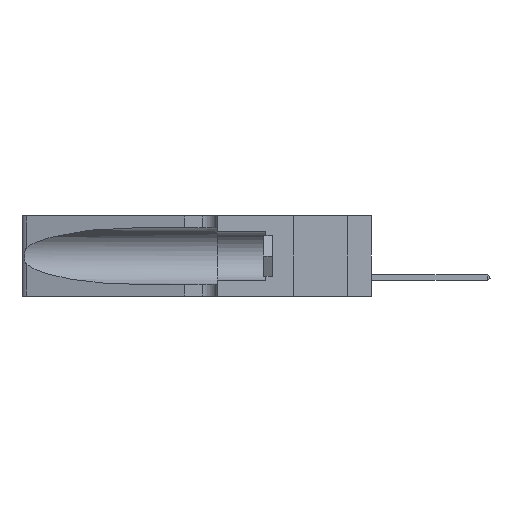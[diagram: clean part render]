
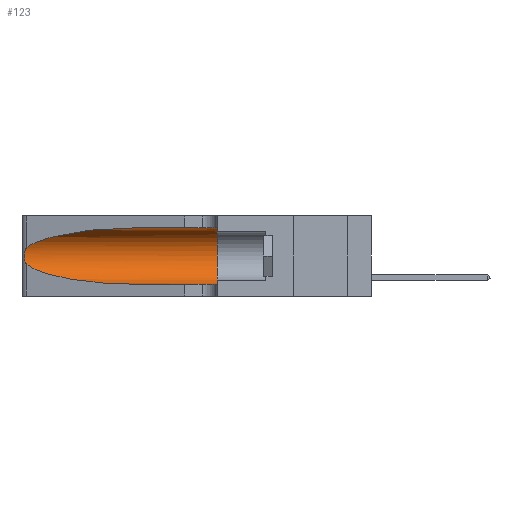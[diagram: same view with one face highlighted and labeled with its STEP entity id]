
A CAD part, left-side view. The second image highlights one B-rep face of the part: STEP entity #123.
In plain terms, the highlighted cylindrical face has radius 3.308 mm (diameter 6.617 mm), a partial arc.
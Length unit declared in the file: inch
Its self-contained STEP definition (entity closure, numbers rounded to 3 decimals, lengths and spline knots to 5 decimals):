
#123 = ADVANCED_FACE ( 'NONE', ( #15983 ), #22076, .F. ) ;
#753 = B_SPLINE_CURVE_WITH_KNOTS ( 'NONE', 3,
 ( #6859, #18631, #8670, #22490, #22673, #6957, #8934, #22578, #10877, #16418, #812, #14480, #6693, #22322 ),
 .UNSPECIFIED., .F., .F.,
 ( 4, 2, 2, 2, 2, 2, 4 ),
 ( 0., 0.00027, 0.00053, 0.00107, 0.0016, 0.00187, 0.00214 ),
 .UNSPECIFIED. ) ;
#812 = CARTESIAN_POINT ( 'NONE',  ( 0.25789, 1.23486, 0.15765 ) ) ;
#2046 = ORIENTED_EDGE ( 'NONE', *, *, #7100, .T. ) ;
#2949 = CARTESIAN_POINT ( 'NONE',  ( 0.25487, 1.22718, 0.14631 ) ) ;
#3954 = EDGE_CURVE ( 'NONE', #23708, #22093, #753, .T. ) ;
#4029 = EDGE_CURVE ( 'NONE', #5796, #17845, #14895, .T. ) ;
#4177 = LINE ( 'NONE', #24890, #17319 ) ;
#4792 = LINE ( 'NONE', #12394, #19177 ) ;
#4969 = CARTESIAN_POINT ( 'NONE',  ( 0.25487, 1.22718, 0.22369 ) ) ;
#5665 = EDGE_LOOP ( 'NONE', ( #6071, #10424, #12598, #2046, #10843, #23635 ) ) ;
#5796 = VERTEX_POINT ( 'NONE', #25244 ) ;
#6071 = ORIENTED_EDGE ( 'NONE', *, *, #22969, .T. ) ;
#6178 = CARTESIAN_POINT ( 'NONE',  ( 0.25487, 1.22718, 0.22369 ) ) ;
#6255 = CARTESIAN_POINT ( 'NONE',  ( 0.18966, 0.96281, 0.31525 ) ) ;
#6427 = CARTESIAN_POINT ( 'NONE',  ( 0.2373, 1.15595, 0.28018 ) ) ;
#6693 = CARTESIAN_POINT ( 'NONE',  ( 0.25555, 1.22993, 0.14849 ) ) ;
#6859 = CARTESIAN_POINT ( 'NONE',  ( 0.25487, 1.22718, 0.22369 ) ) ;
#6957 = CARTESIAN_POINT ( 'NONE',  ( 0.26018, 1.23835, 0.19895 ) ) ;
#7054 = CARTESIAN_POINT ( 'NONE',  ( 0.1305, 1.61858, 0.185 ) ) ;
#7100 = EDGE_CURVE ( 'NONE', #12535, #17845, #4177, .T. ) ;
#8670 = CARTESIAN_POINT ( 'NONE',  ( 0.25639, 1.23184, 0.21858 ) ) ;
#8934 = CARTESIAN_POINT ( 'NONE',  ( 0.26075, 1.23896, 0.19203 ) ) ;
#10037 = CARTESIAN_POINT ( 'NONE',  ( 0.1305, 0.72297, 0.31525 ) ) ;
#10424 = ORIENTED_EDGE ( 'NONE', *, *, #3954, .T. ) ;
#10610 =( BOUNDED_CURVE ( )  B_SPLINE_CURVE ( 3, ( #2949, #22401, #22671, #14885 ),
 .UNSPECIFIED., .F., .F. ) 
 B_SPLINE_CURVE_WITH_KNOTS ( ( 4, 4 ),
 ( 3.44316, 4.71239 ),
 .UNSPECIFIED. ) 
 CURVE ( )  GEOMETRIC_REPRESENTATION_ITEM ( )  RATIONAL_B_SPLINE_CURVE ( ( 1., 0.87, 0.87, 1. ) ) 
 REPRESENTATION_ITEM ( '' )  );
#10843 = ORIENTED_EDGE ( 'NONE', *, *, #4029, .F. ) ;
#10877 = CARTESIAN_POINT ( 'NONE',  ( 0.26017, 1.23833, 0.17102 ) ) ;
#11392 = CARTESIAN_POINT ( 'NONE',  ( 0.1305, 0.72297, 0.31525 ) ) ;
#11445 = AXIS2_PLACEMENT_3D ( 'NONE', #15027, #20889, #17301 ) ;
#11578 = CARTESIAN_POINT ( 'NONE',  ( 0.25487, 1.22718, 0.14631 ) ) ;
#11885 = VERTEX_POINT ( 'NONE', #11392 ) ;
#12394 = CARTESIAN_POINT ( 'NONE',  ( 0.1305, 1.61858, 0.31525 ) ) ;
#12535 = VERTEX_POINT ( 'NONE', #16053 ) ;
#12550 = CARTESIAN_POINT ( 'NONE',  ( 0.1305, 0.35, 0.05475 ) ) ;
#12598 = ORIENTED_EDGE ( 'NONE', *, *, #23451, .T. ) ;
#12937 = DIRECTION ( 'NONE',  ( 0., -1., 0. ) ) ;
#13881 = EDGE_CURVE ( 'NONE', #11885, #5796, #4792, .T. ) ;
#14480 = CARTESIAN_POINT ( 'NONE',  ( 0.25639, 1.23186, 0.15144 ) ) ;
#14885 = CARTESIAN_POINT ( 'NONE',  ( 0.1305, 0.72297, 0.05475 ) ) ;
#14895 = CIRCLE ( 'NONE', #11445, 0.13025 ) ;
#15027 = CARTESIAN_POINT ( 'NONE',  ( 0.1305, 0.35, 0.185 ) ) ;
#15983 = FACE_OUTER_BOUND ( 'NONE', #5665, .T. ) ;
#16053 = CARTESIAN_POINT ( 'NONE',  ( 0.1305, 0.72297, 0.05475 ) ) ;
#16418 = CARTESIAN_POINT ( 'NONE',  ( 0.25856, 1.23593, 0.16098 ) ) ;
#17023 =( BOUNDED_CURVE ( )  B_SPLINE_CURVE ( 3, ( #10037, #6255, #6427, #6178 ),
 .UNSPECIFIED., .F., .T. ) 
 B_SPLINE_CURVE_WITH_KNOTS ( ( 4, 4 ),
 ( 1.5708, 2.84003 ),
 .UNSPECIFIED. ) 
 CURVE ( )  GEOMETRIC_REPRESENTATION_ITEM ( )  RATIONAL_B_SPLINE_CURVE ( ( 1., 0.87, 0.87, 1. ) ) 
 REPRESENTATION_ITEM ( '' )  );
#17301 = DIRECTION ( 'NONE',  ( 0., 0., 1. ) ) ;
#17319 = VECTOR ( 'NONE', #22947, 39.37008 ) ;
#17749 = AXIS2_PLACEMENT_3D ( 'NONE', #7054, #12937, #18471 ) ;
#17845 = VERTEX_POINT ( 'NONE', #12550 ) ;
#18471 = DIRECTION ( 'NONE',  ( 0., 0., -1. ) ) ;
#18631 = CARTESIAN_POINT ( 'NONE',  ( 0.25555, 1.22994, 0.2215 ) ) ;
#19177 = VECTOR ( 'NONE', #21870, 39.37008 ) ;
#20889 = DIRECTION ( 'NONE',  ( 0., 1., 0. ) ) ;
#21870 = DIRECTION ( 'NONE',  ( 0., -1., 0. ) ) ;
#22076 = CYLINDRICAL_SURFACE ( 'NONE', #17749, 0.13025 ) ;
#22093 = VERTEX_POINT ( 'NONE', #11578 ) ;
#22322 = CARTESIAN_POINT ( 'NONE',  ( 0.25487, 1.22718, 0.14631 ) ) ;
#22401 = CARTESIAN_POINT ( 'NONE',  ( 0.2373, 1.15595, 0.08982 ) ) ;
#22490 = CARTESIAN_POINT ( 'NONE',  ( 0.25787, 1.23484, 0.2124 ) ) ;
#22578 = CARTESIAN_POINT ( 'NONE',  ( 0.26075, 1.23896, 0.178 ) ) ;
#22671 = CARTESIAN_POINT ( 'NONE',  ( 0.18966, 0.96281, 0.05475 ) ) ;
#22673 = CARTESIAN_POINT ( 'NONE',  ( 0.25854, 1.2359, 0.20912 ) ) ;
#22947 = DIRECTION ( 'NONE',  ( 0., -1., 0. ) ) ;
#22969 = EDGE_CURVE ( 'NONE', #11885, #23708, #17023, .T. ) ;
#23451 = EDGE_CURVE ( 'NONE', #22093, #12535, #10610, .T. ) ;
#23635 = ORIENTED_EDGE ( 'NONE', *, *, #13881, .F. ) ;
#23708 = VERTEX_POINT ( 'NONE', #4969 ) ;
#24890 = CARTESIAN_POINT ( 'NONE',  ( 0.1305, 1.61858, 0.05475 ) ) ;
#25244 = CARTESIAN_POINT ( 'NONE',  ( 0.1305, 0.35, 0.31525 ) ) ;
